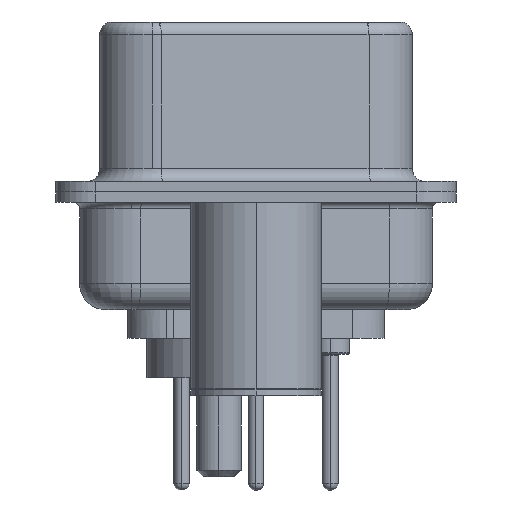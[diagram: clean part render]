
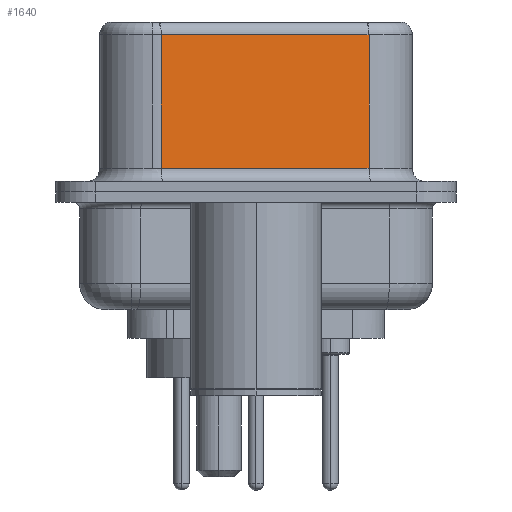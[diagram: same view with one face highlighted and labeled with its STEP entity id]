
A CAD part, left-side view. The second image highlights one B-rep face of the part: STEP entity #1640.
In plain terms, the highlighted planar face has unit normal (-0.985, -0.174, 0).
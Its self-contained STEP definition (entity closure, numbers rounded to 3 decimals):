
#1640 = ADVANCED_FACE ( 'NONE', ( #7983 ), #20477, .F. ) ;
#1793 = ORIENTED_EDGE ( 'NONE', *, *, #20506, .F. ) ;
#2107 = LINE ( 'NONE', #25664, #2889 ) ;
#2169 = CARTESIAN_POINT ( 'NONE',  ( 3.73, 3.628, 6.02 ) ) ;
#2270 = ORIENTED_EDGE ( 'NONE', *, *, #11146, .T. ) ;
#2688 = CARTESIAN_POINT ( 'NONE',  ( 3.73, 3.628, 0.9 ) ) ;
#2709 = EDGE_LOOP ( 'NONE', ( #1793, #2270, #12939, #3487 ) ) ;
#2889 = VECTOR ( 'NONE', #9303, 1000. ) ;
#3421 = VERTEX_POINT ( 'NONE', #12071 ) ;
#3487 = ORIENTED_EDGE ( 'NONE', *, *, #6794, .T. ) ;
#6139 = VECTOR ( 'NONE', #6826, 1000. ) ;
#6794 = EDGE_CURVE ( 'NONE', #7773, #12411, #30294, .T. ) ;
#6826 = DIRECTION ( 'NONE',  ( 0.174, -0.985, 0. ) ) ;
#7543 = DIRECTION ( 'NONE',  ( 0., 0., -1. ) ) ;
#7773 = VERTEX_POINT ( 'NONE', #2688 ) ;
#7983 = FACE_OUTER_BOUND ( 'NONE', #2709, .T. ) ;
#9303 = DIRECTION ( 'NONE',  ( 0., 0., -1. ) ) ;
#9339 = CARTESIAN_POINT ( 'NONE',  ( 5.132, -4.322, 6.02 ) ) ;
#11146 = EDGE_CURVE ( 'NONE', #3421, #16080, #14027, .T. ) ;
#11801 = VECTOR ( 'NONE', #30308, 1000. ) ;
#12071 = CARTESIAN_POINT ( 'NONE',  ( 5.132, -4.322, 6.02 ) ) ;
#12411 = VERTEX_POINT ( 'NONE', #20650 ) ;
#12494 = EDGE_CURVE ( 'NONE', #16080, #7773, #2107, .T. ) ;
#12939 = ORIENTED_EDGE ( 'NONE', *, *, #12494, .T. ) ;
#13490 = AXIS2_PLACEMENT_3D ( 'NONE', #15990, #30504, #29041 ) ;
#14027 = LINE ( 'NONE', #9339, #11801 ) ;
#14645 = CARTESIAN_POINT ( 'NONE',  ( 5.132, -4.322, 0.9 ) ) ;
#15990 = CARTESIAN_POINT ( 'NONE',  ( 5.132, -4.322, 6.52 ) ) ;
#16080 = VERTEX_POINT ( 'NONE', #2169 ) ;
#20477 = PLANE ( 'NONE',  #13490 ) ;
#20506 = EDGE_CURVE ( 'NONE', #3421, #12411, #23024, .T. ) ;
#20650 = CARTESIAN_POINT ( 'NONE',  ( 5.132, -4.322, 0.9 ) ) ;
#22302 = VECTOR ( 'NONE', #7543, 1000. ) ;
#23024 = LINE ( 'NONE', #26270, #22302 ) ;
#25664 = CARTESIAN_POINT ( 'NONE',  ( 3.73, 3.628, 6.52 ) ) ;
#26270 = CARTESIAN_POINT ( 'NONE',  ( 5.132, -4.322, 6.52 ) ) ;
#29041 = DIRECTION ( 'NONE',  ( -0.174, 0.985, 0. ) ) ;
#30294 = LINE ( 'NONE', #14645, #6139 ) ;
#30308 = DIRECTION ( 'NONE',  ( -0.174, 0.985, 0. ) ) ;
#30504 = DIRECTION ( 'NONE',  ( 0.985, 0.174, 0. ) ) ;
